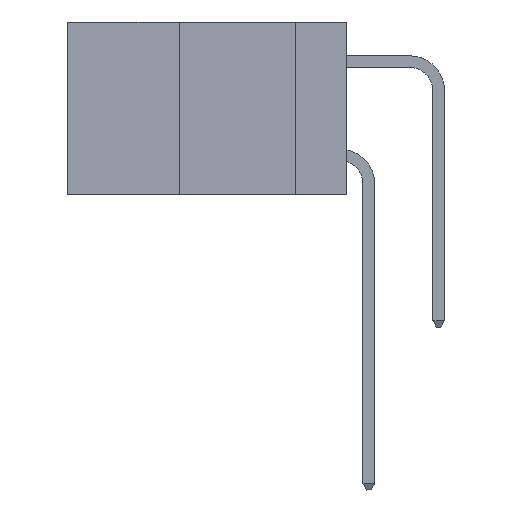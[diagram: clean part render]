
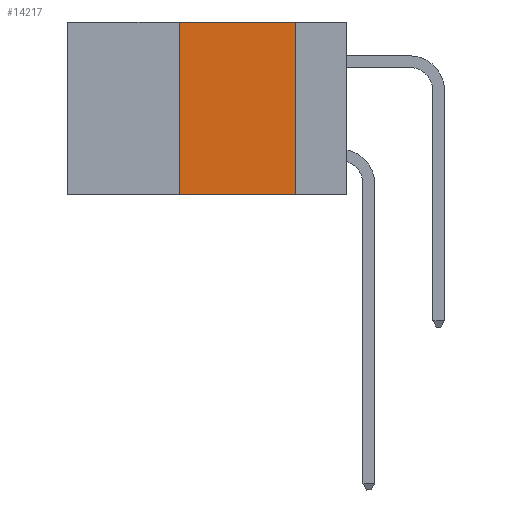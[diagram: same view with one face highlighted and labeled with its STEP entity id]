
A CAD part, left-side view. The second image highlights one B-rep face of the part: STEP entity #14217.
In plain terms, the highlighted planar face has unit normal (-1, 0, 0).
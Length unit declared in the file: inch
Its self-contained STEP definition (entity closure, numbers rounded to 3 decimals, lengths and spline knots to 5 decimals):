
#967 = ORIENTED_EDGE ( 'NONE', *, *, #9638, .F. ) ;
#2854 = CARTESIAN_POINT ( 'NONE',  ( 0., 0.6, 0. ) ) ;
#3110 = AXIS2_PLACEMENT_3D ( 'NONE', #2854, #15347, #4678 ) ;
#4554 = EDGE_CURVE ( 'NONE', #17451, #11795, #22914, .T. ) ;
#4678 = DIRECTION ( 'NONE',  ( 0., 0., -1. ) ) ;
#4755 = EDGE_CURVE ( 'NONE', #17451, #22524, #8153, .T. ) ;
#5047 = CARTESIAN_POINT ( 'NONE',  ( 0., 0.11, 0. ) ) ;
#5828 = ORIENTED_EDGE ( 'NONE', *, *, #10265, .F. ) ;
#6344 = VECTOR ( 'NONE', #8462, 39.37008 ) ;
#6850 = DIRECTION ( 'NONE',  ( 0., 0., -1. ) ) ;
#7239 = CARTESIAN_POINT ( 'NONE',  ( 0., 0.36, -0.37 ) ) ;
#7244 = EDGE_LOOP ( 'NONE', ( #967, #5828, #15838, #20423 ) ) ;
#7578 = VECTOR ( 'NONE', #16821, 39.37008 ) ;
#7716 = CARTESIAN_POINT ( 'NONE',  ( 0., 0.11, 0. ) ) ;
#8153 = LINE ( 'NONE', #21877, #7578 ) ;
#8462 = DIRECTION ( 'NONE',  ( 0., -1., 0. ) ) ;
#9638 = EDGE_CURVE ( 'NONE', #15138, #22524, #10292, .T. ) ;
#10265 = EDGE_CURVE ( 'NONE', #11795, #15138, #11108, .T. ) ;
#10292 = LINE ( 'NONE', #5047, #13938 ) ;
#11108 = LINE ( 'NONE', #20739, #6344 ) ;
#11795 = VERTEX_POINT ( 'NONE', #14649 ) ;
#11804 = PLANE ( 'NONE',  #3110 ) ;
#13938 = VECTOR ( 'NONE', #6850, 39.37008 ) ;
#14217 = ADVANCED_FACE ( 'NONE', ( #21140 ), #11804, .F. ) ;
#14649 = CARTESIAN_POINT ( 'NONE',  ( 0., 0.36, 0. ) ) ;
#15138 = VERTEX_POINT ( 'NONE', #7716 ) ;
#15347 = DIRECTION ( 'NONE',  ( 1., 0., 0. ) ) ;
#15838 = ORIENTED_EDGE ( 'NONE', *, *, #4554, .F. ) ;
#16821 = DIRECTION ( 'NONE',  ( 0., -1., 0. ) ) ;
#17451 = VERTEX_POINT ( 'NONE', #7239 ) ;
#18040 = CARTESIAN_POINT ( 'NONE',  ( 0., 0.36, 0. ) ) ;
#20423 = ORIENTED_EDGE ( 'NONE', *, *, #4755, .T. ) ;
#20739 = CARTESIAN_POINT ( 'NONE',  ( 0., 0.6, 0. ) ) ;
#21086 = CARTESIAN_POINT ( 'NONE',  ( 0., 0.11, -0.37 ) ) ;
#21140 = FACE_OUTER_BOUND ( 'NONE', #7244, .T. ) ;
#21320 = VECTOR ( 'NONE', #21447, 39.37008 ) ;
#21447 = DIRECTION ( 'NONE',  ( 0., 0., 1. ) ) ;
#21877 = CARTESIAN_POINT ( 'NONE',  ( 0., 0.6, -0.37 ) ) ;
#22524 = VERTEX_POINT ( 'NONE', #21086 ) ;
#22914 = LINE ( 'NONE', #18040, #21320 ) ;
